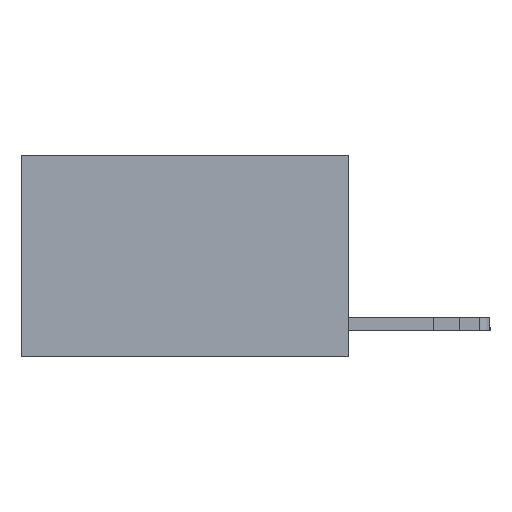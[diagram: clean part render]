
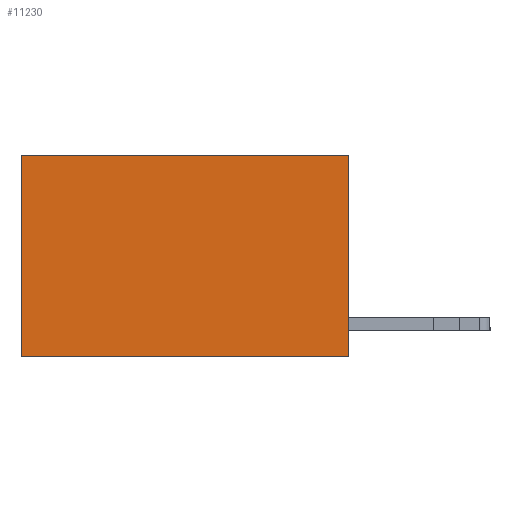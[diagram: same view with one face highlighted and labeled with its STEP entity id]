
A CAD part, left-side view. The second image highlights one B-rep face of the part: STEP entity #11230.
In plain terms, the highlighted planar face has unit normal (-1, 0, 0).
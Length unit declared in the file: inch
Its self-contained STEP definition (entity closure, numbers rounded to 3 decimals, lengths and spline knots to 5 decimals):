
#49 = VECTOR ( 'NONE', #13513, 39.37008 ) ;
#68 = CARTESIAN_POINT ( 'NONE',  ( 0.2625, 0.6, -0.37 ) ) ;
#628 = CARTESIAN_POINT ( 'NONE',  ( 0.2625, 0., -0.37 ) ) ;
#984 = FACE_OUTER_BOUND ( 'NONE', #19455, .T. ) ;
#1305 = DIRECTION ( 'NONE',  ( 1., 0., 0. ) ) ;
#2780 = DIRECTION ( 'NONE',  ( 0., 0., -1. ) ) ;
#3410 = VECTOR ( 'NONE', #10974, 39.37008 ) ;
#3881 = ORIENTED_EDGE ( 'NONE', *, *, #8177, .T. ) ;
#4199 = CARTESIAN_POINT ( 'NONE',  ( 0.2625, 0.6, 0. ) ) ;
#4991 = AXIS2_PLACEMENT_3D ( 'NONE', #19877, #1305, #2780 ) ;
#5062 = CARTESIAN_POINT ( 'NONE',  ( 0.2625, 0., -0.37 ) ) ;
#6386 = VERTEX_POINT ( 'NONE', #5062 ) ;
#7273 = CARTESIAN_POINT ( 'NONE',  ( 0.2625, 0., 0. ) ) ;
#7338 = PLANE ( 'NONE',  #4991 ) ;
#7775 = VERTEX_POINT ( 'NONE', #7273 ) ;
#8177 = EDGE_CURVE ( 'NONE', #17474, #9893, #15780, .T. ) ;
#8380 = CARTESIAN_POINT ( 'NONE',  ( 0.2625, 0.6, 0. ) ) ;
#9893 = VERTEX_POINT ( 'NONE', #68 ) ;
#9940 = ORIENTED_EDGE ( 'NONE', *, *, #11873, .F. ) ;
#9943 = VECTOR ( 'NONE', #12098, 39.37008 ) ;
#10802 = EDGE_CURVE ( 'NONE', #7775, #17474, #18652, .T. ) ;
#10974 = DIRECTION ( 'NONE',  ( 0., 0., -1. ) ) ;
#11230 = ADVANCED_FACE ( 'NONE', ( #984 ), #7338, .F. ) ;
#11873 = EDGE_CURVE ( 'NONE', #7775, #6386, #18045, .T. ) ;
#12098 = DIRECTION ( 'NONE',  ( 0., 1., 0. ) ) ;
#12946 = ORIENTED_EDGE ( 'NONE', *, *, #10802, .T. ) ;
#13271 = VECTOR ( 'NONE', #17965, 39.37008 ) ;
#13513 = DIRECTION ( 'NONE',  ( 0., 0., -1. ) ) ;
#14770 = LINE ( 'NONE', #628, #13271 ) ;
#14969 = CARTESIAN_POINT ( 'NONE',  ( 0.2625, 0., 0. ) ) ;
#15576 = CARTESIAN_POINT ( 'NONE',  ( 0.2625, 0., 0. ) ) ;
#15780 = LINE ( 'NONE', #8380, #3410 ) ;
#16656 = EDGE_CURVE ( 'NONE', #6386, #9893, #14770, .T. ) ;
#16835 = ORIENTED_EDGE ( 'NONE', *, *, #16656, .F. ) ;
#17474 = VERTEX_POINT ( 'NONE', #4199 ) ;
#17965 = DIRECTION ( 'NONE',  ( 0., 1., 0. ) ) ;
#18045 = LINE ( 'NONE', #14969, #49 ) ;
#18652 = LINE ( 'NONE', #15576, #9943 ) ;
#19455 = EDGE_LOOP ( 'NONE', ( #3881, #16835, #9940, #12946 ) ) ;
#19877 = CARTESIAN_POINT ( 'NONE',  ( 0.2625, 0., 0. ) ) ;
